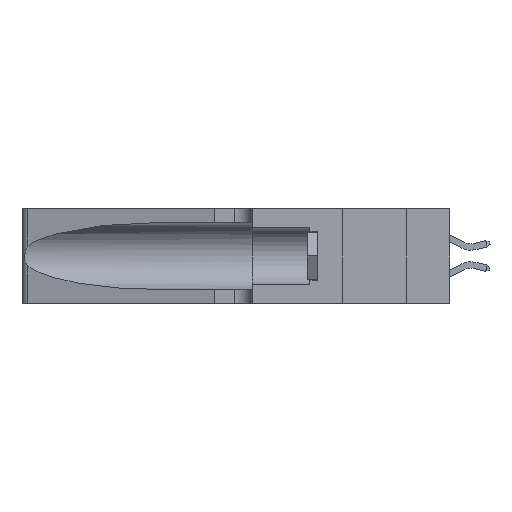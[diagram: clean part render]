
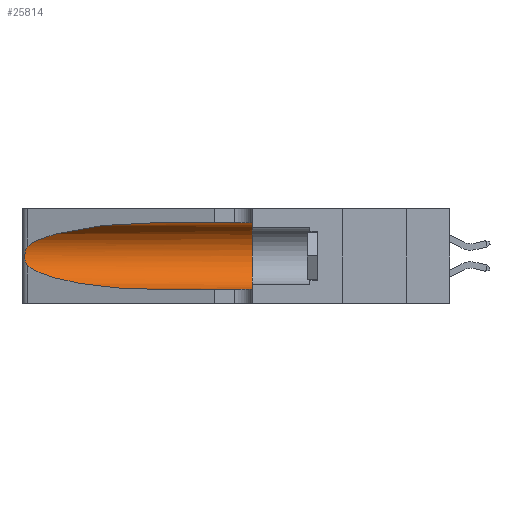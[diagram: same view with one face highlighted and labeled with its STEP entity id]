
A CAD part, left-side view. The second image highlights one B-rep face of the part: STEP entity #25814.
In plain terms, the highlighted cylindrical face has radius 3.308 mm (diameter 6.617 mm), a partial arc.
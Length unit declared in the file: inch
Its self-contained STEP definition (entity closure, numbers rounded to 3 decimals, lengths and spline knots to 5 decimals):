
#190 = FACE_OUTER_BOUND ( 'NONE', #9586, .T. ) ;
#994 = EDGE_CURVE ( 'NONE', #38958, #42426, #3152, .T. ) ;
#2664 = ORIENTED_EDGE ( 'NONE', *, *, #24122, .F. ) ;
#3152 =( BOUNDED_CURVE ( )  B_SPLINE_CURVE ( 3, ( #32664, #6359, #26110, #13096 ),
 .UNSPECIFIED., .F., .F. ) 
 B_SPLINE_CURVE_WITH_KNOTS ( ( 4, 4 ),
 ( 1.5708, 2.84003 ),
 .UNSPECIFIED. ) 
 CURVE ( )  GEOMETRIC_REPRESENTATION_ITEM ( )  RATIONAL_B_SPLINE_CURVE ( ( 1., 0.87, 0.87, 1. ) ) 
 REPRESENTATION_ITEM ( '' )  );
#3161 = CARTESIAN_POINT ( 'NONE',  ( 0.25787, 1.23484, 0.2124 ) ) ;
#3175 = VERTEX_POINT ( 'NONE', #30645 ) ;
#3203 = ORIENTED_EDGE ( 'NONE', *, *, #27941, .T. ) ;
#3280 = VERTEX_POINT ( 'NONE', #37628 ) ;
#3749 = CARTESIAN_POINT ( 'NONE',  ( 0.1305, 0.35, 0.05475 ) ) ;
#6359 = CARTESIAN_POINT ( 'NONE',  ( 0.18966, 0.96281, 0.31525 ) ) ;
#6510 = CARTESIAN_POINT ( 'NONE',  ( 0.26018, 1.23835, 0.19895 ) ) ;
#6842 = ORIENTED_EDGE ( 'NONE', *, *, #41575, .T. ) ;
#7171 = AXIS2_PLACEMENT_3D ( 'NONE', #15238, #38088, #18513 ) ;
#8412 = CARTESIAN_POINT ( 'NONE',  ( 0.25487, 1.22718, 0.22369 ) ) ;
#9586 = EDGE_LOOP ( 'NONE', ( #25938, #3203, #34080, #6842, #2664, #18185 ) ) ;
#9886 = CARTESIAN_POINT ( 'NONE',  ( 0.26075, 1.23896, 0.178 ) ) ;
#9893 = CARTESIAN_POINT ( 'NONE',  ( 0.1305, 0.72297, 0.31525 ) ) ;
#13096 = CARTESIAN_POINT ( 'NONE',  ( 0.25487, 1.22718, 0.22369 ) ) ;
#13251 = CARTESIAN_POINT ( 'NONE',  ( 0.25856, 1.23593, 0.16098 ) ) ;
#14650 = CARTESIAN_POINT ( 'NONE',  ( 0.1305, 1.61858, 0.31525 ) ) ;
#15238 = CARTESIAN_POINT ( 'NONE',  ( 0.1305, 0.35, 0.185 ) ) ;
#15378 = CARTESIAN_POINT ( 'NONE',  ( 0.1305, 1.61858, 0.185 ) ) ;
#16378 = CARTESIAN_POINT ( 'NONE',  ( 0.25487, 1.22718, 0.22369 ) ) ;
#16511 = CARTESIAN_POINT ( 'NONE',  ( 0.25639, 1.23186, 0.15144 ) ) ;
#16799 = VECTOR ( 'NONE', #39436, 39.37008 ) ;
#18185 = ORIENTED_EDGE ( 'NONE', *, *, #28548, .F. ) ;
#18513 = DIRECTION ( 'NONE',  ( 0., 0., 1. ) ) ;
#19471 = LINE ( 'NONE', #14650, #27160 ) ;
#19802 = CARTESIAN_POINT ( 'NONE',  ( 0.25487, 1.22718, 0.14631 ) ) ;
#19867 = B_SPLINE_CURVE_WITH_KNOTS ( 'NONE', 3,
 ( #16378, #42534, #22960, #3161, #26257, #6510, #29523, #9886, #32815, #13251, #36089, #16511, #39374, #19802 ),
 .UNSPECIFIED., .F., .F.,
 ( 4, 2, 2, 2, 2, 2, 4 ),
 ( 0., 0.00027, 0.00053, 0.00107, 0.0016, 0.00187, 0.00214 ),
 .UNSPECIFIED. ) ;
#20485 = CARTESIAN_POINT ( 'NONE',  ( 0.1305, 0.72297, 0.05475 ) ) ;
#22960 = CARTESIAN_POINT ( 'NONE',  ( 0.25639, 1.23184, 0.21858 ) ) ;
#24122 = EDGE_CURVE ( 'NONE', #3280, #33490, #30578, .T. ) ;
#24320 =( BOUNDED_CURVE ( )  B_SPLINE_CURVE ( 3, ( #36773, #33479, #40039, #20485 ),
 .UNSPECIFIED., .F., .T. ) 
 B_SPLINE_CURVE_WITH_KNOTS ( ( 4, 4 ),
 ( 3.44316, 4.71239 ),
 .UNSPECIFIED. ) 
 CURVE ( )  GEOMETRIC_REPRESENTATION_ITEM ( )  RATIONAL_B_SPLINE_CURVE ( ( 1., 0.87, 0.87, 1. ) ) 
 REPRESENTATION_ITEM ( '' )  );
#25399 = CYLINDRICAL_SURFACE ( 'NONE', #25727, 0.13025 ) ;
#25727 = AXIS2_PLACEMENT_3D ( 'NONE', #15378, #28381, #38231 ) ;
#25814 = ADVANCED_FACE ( 'NONE', ( #190 ), #25399, .F. ) ;
#25938 = ORIENTED_EDGE ( 'NONE', *, *, #994, .T. ) ;
#26110 = CARTESIAN_POINT ( 'NONE',  ( 0.2373, 1.15595, 0.28018 ) ) ;
#26257 = CARTESIAN_POINT ( 'NONE',  ( 0.25854, 1.2359, 0.20912 ) ) ;
#26672 = VERTEX_POINT ( 'NONE', #35765 ) ;
#27160 = VECTOR ( 'NONE', #40778, 39.37008 ) ;
#27941 = EDGE_CURVE ( 'NONE', #42426, #3175, #19867, .T. ) ;
#28381 = DIRECTION ( 'NONE',  ( 0., -1., 0. ) ) ;
#28548 = EDGE_CURVE ( 'NONE', #38958, #3280, #19471, .T. ) ;
#29523 = CARTESIAN_POINT ( 'NONE',  ( 0.26075, 1.23896, 0.19203 ) ) ;
#30578 = CIRCLE ( 'NONE', #7171, 0.13025 ) ;
#30645 = CARTESIAN_POINT ( 'NONE',  ( 0.25487, 1.22718, 0.14631 ) ) ;
#32664 = CARTESIAN_POINT ( 'NONE',  ( 0.1305, 0.72297, 0.31525 ) ) ;
#32815 = CARTESIAN_POINT ( 'NONE',  ( 0.26017, 1.23833, 0.17102 ) ) ;
#33479 = CARTESIAN_POINT ( 'NONE',  ( 0.2373, 1.15595, 0.08982 ) ) ;
#33490 = VERTEX_POINT ( 'NONE', #3749 ) ;
#34080 = ORIENTED_EDGE ( 'NONE', *, *, #37752, .T. ) ;
#34186 = LINE ( 'NONE', #36146, #16799 ) ;
#35765 = CARTESIAN_POINT ( 'NONE',  ( 0.1305, 0.72297, 0.05475 ) ) ;
#36089 = CARTESIAN_POINT ( 'NONE',  ( 0.25789, 1.23486, 0.15765 ) ) ;
#36146 = CARTESIAN_POINT ( 'NONE',  ( 0.1305, 1.61858, 0.05475 ) ) ;
#36773 = CARTESIAN_POINT ( 'NONE',  ( 0.25487, 1.22718, 0.14631 ) ) ;
#37628 = CARTESIAN_POINT ( 'NONE',  ( 0.1305, 0.35, 0.31525 ) ) ;
#37752 = EDGE_CURVE ( 'NONE', #3175, #26672, #24320, .T. ) ;
#38088 = DIRECTION ( 'NONE',  ( 0., 1., 0. ) ) ;
#38231 = DIRECTION ( 'NONE',  ( 0., 0., -1. ) ) ;
#38958 = VERTEX_POINT ( 'NONE', #9893 ) ;
#39374 = CARTESIAN_POINT ( 'NONE',  ( 0.25555, 1.22993, 0.14849 ) ) ;
#39436 = DIRECTION ( 'NONE',  ( 0., -1., 0. ) ) ;
#40039 = CARTESIAN_POINT ( 'NONE',  ( 0.18966, 0.96281, 0.05475 ) ) ;
#40778 = DIRECTION ( 'NONE',  ( 0., -1., 0. ) ) ;
#41575 = EDGE_CURVE ( 'NONE', #26672, #33490, #34186, .T. ) ;
#42426 = VERTEX_POINT ( 'NONE', #8412 ) ;
#42534 = CARTESIAN_POINT ( 'NONE',  ( 0.25555, 1.22994, 0.2215 ) ) ;
